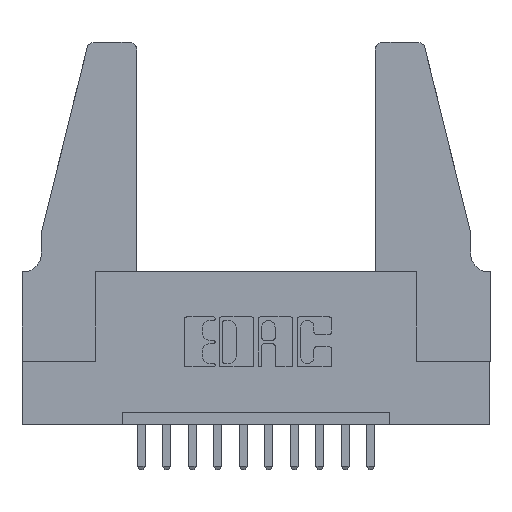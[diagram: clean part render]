
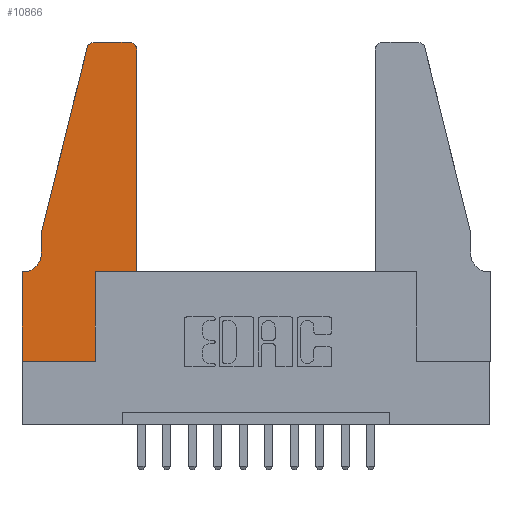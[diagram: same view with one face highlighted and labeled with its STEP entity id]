
A CAD part, top view. The second image highlights one B-rep face of the part: STEP entity #10866.
In plain terms, the highlighted planar face has unit normal (0, 0, 1).
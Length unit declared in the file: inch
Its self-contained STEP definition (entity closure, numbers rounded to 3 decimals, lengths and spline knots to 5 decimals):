
#58 = CARTESIAN_POINT ( 'NONE',  ( 0.284, 1.25, 0.37 ) ) ;
#78 = LINE ( 'NONE', #4338, #10998 ) ;
#168 = DIRECTION ( 'NONE',  ( 1., 0., 0. ) ) ;
#277 = VERTEX_POINT ( 'NONE', #9112 ) ;
#394 = VERTEX_POINT ( 'NONE', #5670 ) ;
#447 = CARTESIAN_POINT ( 'NONE',  ( 0.2865, 0., 0.37 ) ) ;
#678 = PLANE ( 'NONE',  #7105 ) ;
#774 = LINE ( 'NONE', #12718, #9627 ) ;
#777 = DIRECTION ( 'NONE',  ( 1., 0., 0. ) ) ;
#792 = DIRECTION ( 'NONE',  ( 1., 0., 0. ) ) ;
#1079 = DIRECTION ( 'NONE',  ( 0., 1., 0. ) ) ;
#1131 = EDGE_CURVE ( 'NONE', #13932, #12378, #14074, .T. ) ;
#1212 = CARTESIAN_POINT ( 'NONE',  ( 0., 0., 0.37 ) ) ;
#1230 = DIRECTION ( 'NONE',  ( 0., -1., 0. ) ) ;
#1812 = CARTESIAN_POINT ( 'NONE',  ( 0., 0.35, 0.37 ) ) ;
#1981 = DIRECTION ( 'NONE',  ( 1., 0., 0. ) ) ;
#1985 = DIRECTION ( 'NONE',  ( 0., 1., 0. ) ) ;
#2260 = VERTEX_POINT ( 'NONE', #11195 ) ;
#2578 = EDGE_CURVE ( 'NONE', #13173, #277, #6524, .T. ) ;
#3005 = ORIENTED_EDGE ( 'NONE', *, *, #5679, .T. ) ;
#3378 = VERTEX_POINT ( 'NONE', #58 ) ;
#3586 = ORIENTED_EDGE ( 'NONE', *, *, #11281, .T. ) ;
#3696 = CARTESIAN_POINT ( 'NONE',  ( 0.0755, 0.5, 0.37 ) ) ;
#3716 = VECTOR ( 'NONE', #7577, 39.37008 ) ;
#3794 = EDGE_CURVE ( 'NONE', #3378, #13537, #12765, .T. ) ;
#3894 = ORIENTED_EDGE ( 'NONE', *, *, #10463, .T. ) ;
#4017 = VECTOR ( 'NONE', #7889, 39.37008 ) ;
#4194 = CARTESIAN_POINT ( 'NONE',  ( 0.25487, 1.22718, 0.37 ) ) ;
#4204 = VERTEX_POINT ( 'NONE', #447 ) ;
#4338 = CARTESIAN_POINT ( 'NONE',  ( 0.2605, 1.25, 0.37 ) ) ;
#4533 = DIRECTION ( 'NONE',  ( -1., 0., 0. ) ) ;
#5218 = DIRECTION ( 'NONE',  ( 0., 0., 1. ) ) ;
#5262 = EDGE_LOOP ( 'NONE', ( #13747, #9029, #8364, #8114, #6346, #8681, #12604, #3894, #9897, #3586, #11114, #3005 ) ) ;
#5489 = CARTESIAN_POINT ( 'NONE',  ( 0.2865, 0.35, 0.37 ) ) ;
#5506 = CARTESIAN_POINT ( 'NONE',  ( 0., 0., 0.37 ) ) ;
#5670 = CARTESIAN_POINT ( 'NONE',  ( 0.2865, 0.35, 0.37 ) ) ;
#5679 = EDGE_CURVE ( 'NONE', #277, #2260, #12491, .T. ) ;
#5787 = EDGE_CURVE ( 'NONE', #13537, #13667, #774, .T. ) ;
#5791 = EDGE_CURVE ( 'NONE', #2260, #3378, #78, .T. ) ;
#6123 = DIRECTION ( 'NONE',  ( -0.239, -0.971, 0. ) ) ;
#6213 = CARTESIAN_POINT ( 'NONE',  ( 0.4205, 1.22, 0.37 ) ) ;
#6346 = ORIENTED_EDGE ( 'NONE', *, *, #9703, .T. ) ;
#6414 = CARTESIAN_POINT ( 'NONE',  ( 0.4505, 0.35, 0.37 ) ) ;
#6519 = LINE ( 'NONE', #9907, #13819 ) ;
#6524 = LINE ( 'NONE', #6414, #11638 ) ;
#6980 = CARTESIAN_POINT ( 'NONE',  ( 0.0755, 0.42, 0.37 ) ) ;
#7043 = CARTESIAN_POINT ( 'NONE',  ( 0.0055, 0.35, 0.37 ) ) ;
#7105 = AXIS2_PLACEMENT_3D ( 'NONE', #1812, #8307, #777 ) ;
#7313 = EDGE_CURVE ( 'NONE', #13667, #9008, #6519, .T. ) ;
#7328 = DIRECTION ( 'NONE',  ( 0., 0., 1. ) ) ;
#7500 = CARTESIAN_POINT ( 'NONE',  ( 0.4505, 0.35, 0.37 ) ) ;
#7577 = DIRECTION ( 'NONE',  ( -1., 0., 0. ) ) ;
#7824 = FACE_OUTER_BOUND ( 'NONE', #5262, .T. ) ;
#7889 = DIRECTION ( 'NONE',  ( 0., -1., 0. ) ) ;
#8114 = ORIENTED_EDGE ( 'NONE', *, *, #7313, .T. ) ;
#8307 = DIRECTION ( 'NONE',  ( 0., 0., 1. ) ) ;
#8364 = ORIENTED_EDGE ( 'NONE', *, *, #5787, .T. ) ;
#8516 = AXIS2_PLACEMENT_3D ( 'NONE', #9561, #5218, #1981 ) ;
#8586 = CARTESIAN_POINT ( 'NONE',  ( 0.4505, 0.35, 0.37 ) ) ;
#8681 = ORIENTED_EDGE ( 'NONE', *, *, #10552, .T. ) ;
#8884 = AXIS2_PLACEMENT_3D ( 'NONE', #6213, #7328, #792 ) ;
#9008 = VERTEX_POINT ( 'NONE', #6980 ) ;
#9029 = ORIENTED_EDGE ( 'NONE', *, *, #3794, .T. ) ;
#9112 = CARTESIAN_POINT ( 'NONE',  ( 0.4505, 1.22, 0.37 ) ) ;
#9439 = AXIS2_PLACEMENT_3D ( 'NONE', #11060, #13237, #4533 ) ;
#9561 = CARTESIAN_POINT ( 'NONE',  ( 0.284, 1.22, 0.37 ) ) ;
#9621 = DIRECTION ( 'NONE',  ( -1., 0., 0. ) ) ;
#9627 = VECTOR ( 'NONE', #6123, 39.37008 ) ;
#9703 = EDGE_CURVE ( 'NONE', #9008, #10227, #9711, .T. ) ;
#9711 = CIRCLE ( 'NONE', #9439, 0.07 ) ;
#9856 = VECTOR ( 'NONE', #168, 39.37008 ) ;
#9897 = ORIENTED_EDGE ( 'NONE', *, *, #13879, .T. ) ;
#9907 = CARTESIAN_POINT ( 'NONE',  ( 0.0755, 0.5, 0.37 ) ) ;
#10184 = LINE ( 'NONE', #5506, #9856 ) ;
#10227 = VERTEX_POINT ( 'NONE', #7043 ) ;
#10463 = EDGE_CURVE ( 'NONE', #12378, #4204, #10184, .T. ) ;
#10552 = EDGE_CURVE ( 'NONE', #10227, #13932, #11722, .T. ) ;
#10770 = DIRECTION ( 'NONE',  ( 1., 0., 0. ) ) ;
#10866 = ADVANCED_FACE ( 'NONE', ( #7824 ), #678, .T. ) ;
#10998 = VECTOR ( 'NONE', #9621, 39.37008 ) ;
#11060 = CARTESIAN_POINT ( 'NONE',  ( 0.0055, 0.42, 0.37 ) ) ;
#11114 = ORIENTED_EDGE ( 'NONE', *, *, #2578, .T. ) ;
#11195 = CARTESIAN_POINT ( 'NONE',  ( 0.4205, 1.25, 0.37 ) ) ;
#11281 = EDGE_CURVE ( 'NONE', #394, #13173, #13830, .T. ) ;
#11638 = VECTOR ( 'NONE', #1985, 39.37008 ) ;
#11722 = LINE ( 'NONE', #11756, #3716 ) ;
#11735 = VECTOR ( 'NONE', #1079, 39.37008 ) ;
#11756 = CARTESIAN_POINT ( 'NONE',  ( 0.0755, 0.35, 0.37 ) ) ;
#12378 = VERTEX_POINT ( 'NONE', #13386 ) ;
#12398 = LINE ( 'NONE', #5489, #11735 ) ;
#12491 = CIRCLE ( 'NONE', #8884, 0.03 ) ;
#12604 = ORIENTED_EDGE ( 'NONE', *, *, #1131, .T. ) ;
#12718 = CARTESIAN_POINT ( 'NONE',  ( 0.0755, 0.5, 0.37 ) ) ;
#12765 = CIRCLE ( 'NONE', #8516, 0.03 ) ;
#13004 = CARTESIAN_POINT ( 'NONE',  ( 0., 0.35, 0.37 ) ) ;
#13173 = VERTEX_POINT ( 'NONE', #8586 ) ;
#13237 = DIRECTION ( 'NONE',  ( 0., 0., -1. ) ) ;
#13326 = VECTOR ( 'NONE', #10770, 39.37008 ) ;
#13386 = CARTESIAN_POINT ( 'NONE',  ( 0., 0., 0.37 ) ) ;
#13537 = VERTEX_POINT ( 'NONE', #4194 ) ;
#13667 = VERTEX_POINT ( 'NONE', #3696 ) ;
#13747 = ORIENTED_EDGE ( 'NONE', *, *, #5791, .T. ) ;
#13819 = VECTOR ( 'NONE', #1230, 39.37008 ) ;
#13830 = LINE ( 'NONE', #7500, #13326 ) ;
#13879 = EDGE_CURVE ( 'NONE', #4204, #394, #12398, .T. ) ;
#13932 = VERTEX_POINT ( 'NONE', #13004 ) ;
#14074 = LINE ( 'NONE', #1212, #4017 ) ;
